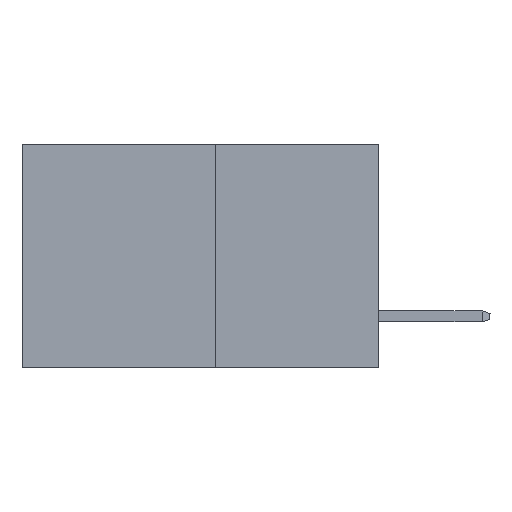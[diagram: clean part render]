
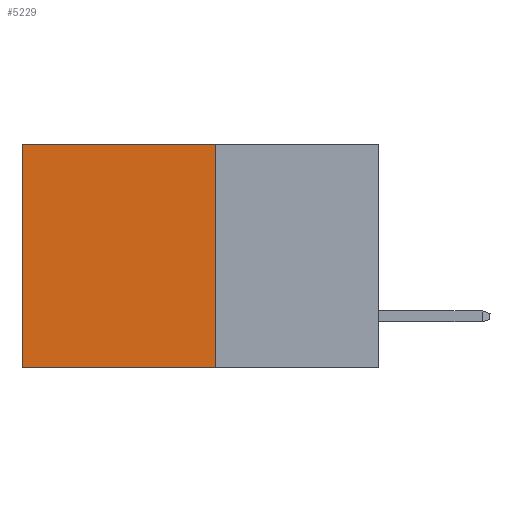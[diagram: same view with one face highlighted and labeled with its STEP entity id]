
A CAD part, left-side view. The second image highlights one B-rep face of the part: STEP entity #5229.
In plain terms, the highlighted planar face has unit normal (-1, 0, 0).
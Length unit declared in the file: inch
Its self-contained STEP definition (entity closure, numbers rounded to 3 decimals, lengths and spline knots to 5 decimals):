
#336 = DIRECTION ( 'NONE',  ( 0., 0., -1. ) ) ;
#997 = ORIENTED_EDGE ( 'NONE', *, *, #6628, .F. ) ;
#1138 = VECTOR ( 'NONE', #7722, 39.37008 ) ;
#2881 = VECTOR ( 'NONE', #26653, 39.37008 ) ;
#3438 = ORIENTED_EDGE ( 'NONE', *, *, #3615, .T. ) ;
#3615 = EDGE_CURVE ( 'NONE', #18379, #16913, #10151, .T. ) ;
#5086 = AXIS2_PLACEMENT_3D ( 'NONE', #12205, #25037, #25430 ) ;
#5229 = ADVANCED_FACE ( 'NONE', ( #6092 ), #25045, .F. ) ;
#6092 = FACE_OUTER_BOUND ( 'NONE', #25064, .T. ) ;
#6628 = EDGE_CURVE ( 'NONE', #17111, #16913, #12585, .T. ) ;
#7054 = VECTOR ( 'NONE', #20766, 39.37008 ) ;
#7722 = DIRECTION ( 'NONE',  ( 0., 1., 0. ) ) ;
#7929 = LINE ( 'NONE', #23577, #1138 ) ;
#8175 = CARTESIAN_POINT ( 'NONE',  ( 0.277, 0.59, -0.37 ) ) ;
#9226 = EDGE_CURVE ( 'NONE', #14927, #18379, #7929, .T. ) ;
#10151 = LINE ( 'NONE', #17518, #21717 ) ;
#12205 = CARTESIAN_POINT ( 'NONE',  ( 0.277, 0.27, -0.37 ) ) ;
#12585 = LINE ( 'NONE', #26756, #7054 ) ;
#13448 = CARTESIAN_POINT ( 'NONE',  ( 0.277, 0.27, -0.37 ) ) ;
#14927 = VERTEX_POINT ( 'NONE', #22095 ) ;
#16913 = VERTEX_POINT ( 'NONE', #8175 ) ;
#17111 = VERTEX_POINT ( 'NONE', #13448 ) ;
#17518 = CARTESIAN_POINT ( 'NONE',  ( 0.277, 0.59, -0.37 ) ) ;
#18379 = VERTEX_POINT ( 'NONE', #20261 ) ;
#20261 = CARTESIAN_POINT ( 'NONE',  ( 0.277, 0.59, 0. ) ) ;
#20766 = DIRECTION ( 'NONE',  ( 0., 1., 0. ) ) ;
#21717 = VECTOR ( 'NONE', #336, 39.37008 ) ;
#22095 = CARTESIAN_POINT ( 'NONE',  ( 0.277, 0.27, 0. ) ) ;
#22632 = ORIENTED_EDGE ( 'NONE', *, *, #9226, .T. ) ;
#23577 = CARTESIAN_POINT ( 'NONE',  ( 0.277, 0.27, 0. ) ) ;
#24148 = EDGE_CURVE ( 'NONE', #14927, #17111, #27231, .T. ) ;
#24397 = CARTESIAN_POINT ( 'NONE',  ( 0.277, 0.27, -0.37 ) ) ;
#25037 = DIRECTION ( 'NONE',  ( 1., 0., 0. ) ) ;
#25045 = PLANE ( 'NONE',  #5086 ) ;
#25064 = EDGE_LOOP ( 'NONE', ( #3438, #997, #29176, #22632 ) ) ;
#25430 = DIRECTION ( 'NONE',  ( 0., 0., -1. ) ) ;
#26653 = DIRECTION ( 'NONE',  ( 0., 0., -1. ) ) ;
#26756 = CARTESIAN_POINT ( 'NONE',  ( 0.277, 0.27, -0.37 ) ) ;
#27231 = LINE ( 'NONE', #24397, #2881 ) ;
#29176 = ORIENTED_EDGE ( 'NONE', *, *, #24148, .F. ) ;
